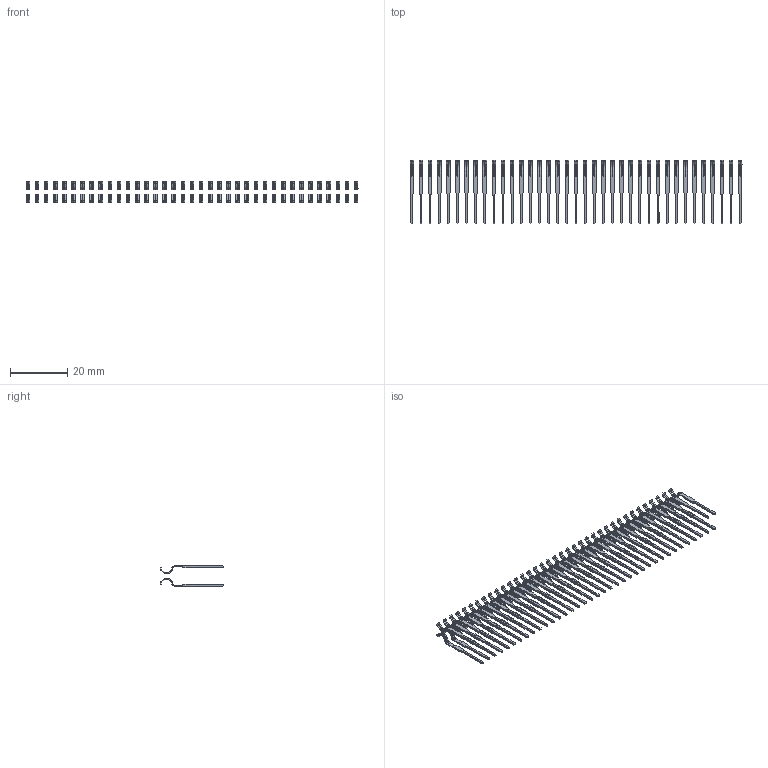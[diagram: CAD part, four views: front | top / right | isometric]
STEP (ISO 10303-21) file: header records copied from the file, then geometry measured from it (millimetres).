
FILE_DESCRIPTION (( 'STEP AP203' ), '1' );
FILE_NAME ('346-074-526-802.STEP', '2022-05-25T02:21:33', ( '' ), ( '' ), 'SwSTEP 2.0', 'SolidWorks 2020', '' );
FILE_SCHEMA (( 'CONFIG_CONTROL_DESIGN' ));
Length unit declared in the file: inch
Products named in the file (3): 345-292-001_345-293-126; 346-074-526-802; 346 Part_0.170 Offset - 0.128 Dia
Assembly tree (75 placements, depth 2):
  346-074-526-802
    346 Part_0.170 Offset - 0.128 Dia
    345-292-001_345-293-126  x74
Bounding box: 115.57 x 22.23 x 6.99 mm (x, y, z)
Volume: 787.2 mm3; surface area: 5465.6 mm2
Topology: 74 solids, 74 shells, 3404 faces, 9916 edges, 6512 vertices
Faces by surface type: plane 2220, cylinder 1184
Entity records: 24973 total; most frequent: CARTESIAN_POINT 4124, ORIENTED_EDGE 4058, DIRECTION 3685, EDGE_CURVE 2029, LINE 1749, VECTOR 1749, VERTEX_POINT 1350, AXIS2_PLACEMENT_3D 968
